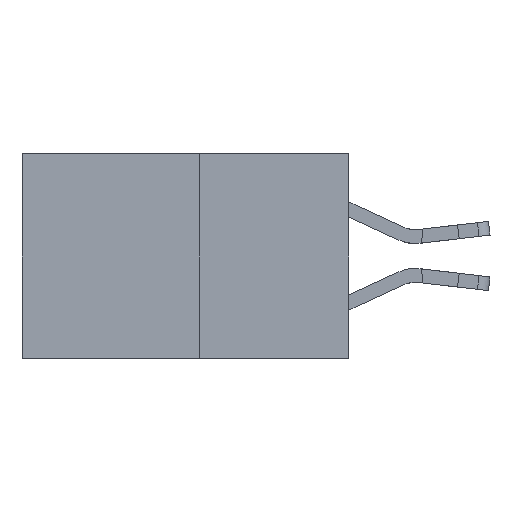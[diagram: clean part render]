
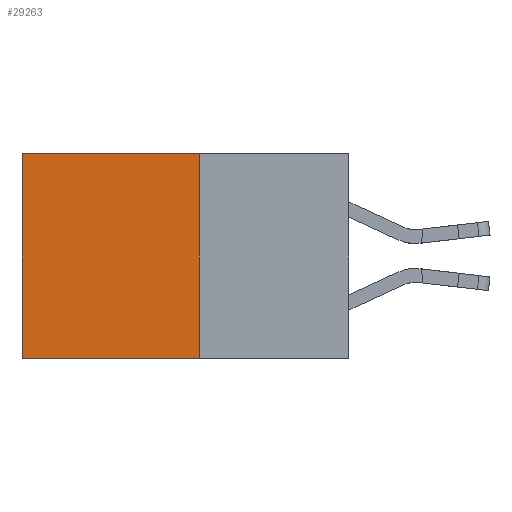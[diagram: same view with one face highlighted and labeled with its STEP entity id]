
A CAD part, left-side view. The second image highlights one B-rep face of the part: STEP entity #29263.
In plain terms, the highlighted planar face has unit normal (-1, 0, 0).
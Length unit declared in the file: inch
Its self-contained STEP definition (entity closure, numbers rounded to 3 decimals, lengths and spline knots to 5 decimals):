
#2054 = ORIENTED_EDGE ( 'NONE', *, *, #22281, .T. ) ;
#2079 = CARTESIAN_POINT ( 'NONE',  ( 0.277, 0.27, -0.37 ) ) ;
#3483 = DIRECTION ( 'NONE',  ( 0., 0., -1. ) ) ;
#3781 = CARTESIAN_POINT ( 'NONE',  ( 0.277, 0.27, -0.37 ) ) ;
#4297 = EDGE_CURVE ( 'NONE', #18095, #16364, #30275, .T. ) ;
#4305 = CARTESIAN_POINT ( 'NONE',  ( 0.277, 0.27, -0.37 ) ) ;
#5635 = VERTEX_POINT ( 'NONE', #23781 ) ;
#5763 = CARTESIAN_POINT ( 'NONE',  ( 0.277, 0.59, -0.37 ) ) ;
#6614 = EDGE_CURVE ( 'NONE', #16364, #14996, #22668, .T. ) ;
#7049 = DIRECTION ( 'NONE',  ( 1., 0., 0. ) ) ;
#8341 = DIRECTION ( 'NONE',  ( 0., 0., -1. ) ) ;
#12634 = CARTESIAN_POINT ( 'NONE',  ( 0.277, 0.27, 0. ) ) ;
#12914 = VECTOR ( 'NONE', #8341, 39.37008 ) ;
#14996 = VERTEX_POINT ( 'NONE', #19588 ) ;
#15577 = ORIENTED_EDGE ( 'NONE', *, *, #6614, .F. ) ;
#16364 = VERTEX_POINT ( 'NONE', #4305 ) ;
#17967 = FACE_OUTER_BOUND ( 'NONE', #23802, .T. ) ;
#18067 = CARTESIAN_POINT ( 'NONE',  ( 0.277, 0.27, 0. ) ) ;
#18095 = VERTEX_POINT ( 'NONE', #18067 ) ;
#19588 = CARTESIAN_POINT ( 'NONE',  ( 0.277, 0.59, -0.37 ) ) ;
#20709 = AXIS2_PLACEMENT_3D ( 'NONE', #29523, #7049, #24592 ) ;
#21981 = VECTOR ( 'NONE', #25194, 39.37008 ) ;
#22281 = EDGE_CURVE ( 'NONE', #18095, #5635, #28661, .T. ) ;
#22668 = LINE ( 'NONE', #2079, #28578 ) ;
#22929 = ORIENTED_EDGE ( 'NONE', *, *, #4297, .F. ) ;
#23591 = VECTOR ( 'NONE', #3483, 39.37008 ) ;
#23751 = EDGE_CURVE ( 'NONE', #5635, #14996, #31261, .T. ) ;
#23781 = CARTESIAN_POINT ( 'NONE',  ( 0.277, 0.59, 0. ) ) ;
#23802 = EDGE_LOOP ( 'NONE', ( #23877, #15577, #22929, #2054 ) ) ;
#23877 = ORIENTED_EDGE ( 'NONE', *, *, #23751, .T. ) ;
#24592 = DIRECTION ( 'NONE',  ( 0., 0., -1. ) ) ;
#25194 = DIRECTION ( 'NONE',  ( 0., 1., 0. ) ) ;
#28578 = VECTOR ( 'NONE', #29771, 39.37008 ) ;
#28661 = LINE ( 'NONE', #12634, #21981 ) ;
#29263 = ADVANCED_FACE ( 'NONE', ( #17967 ), #32024, .F. ) ;
#29523 = CARTESIAN_POINT ( 'NONE',  ( 0.277, 0.27, -0.37 ) ) ;
#29771 = DIRECTION ( 'NONE',  ( 0., 1., 0. ) ) ;
#30275 = LINE ( 'NONE', #3781, #23591 ) ;
#31261 = LINE ( 'NONE', #5763, #12914 ) ;
#32024 = PLANE ( 'NONE',  #20709 ) ;
